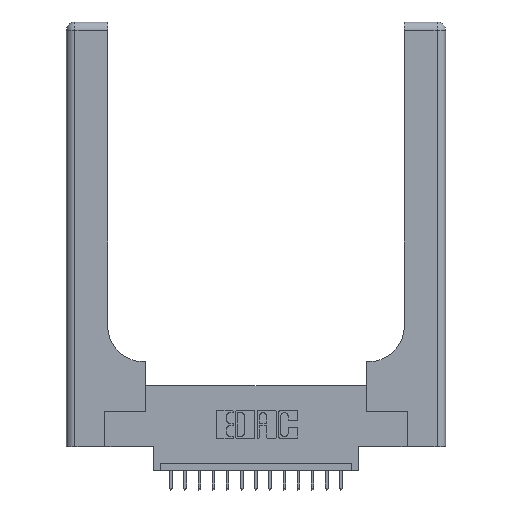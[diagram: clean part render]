
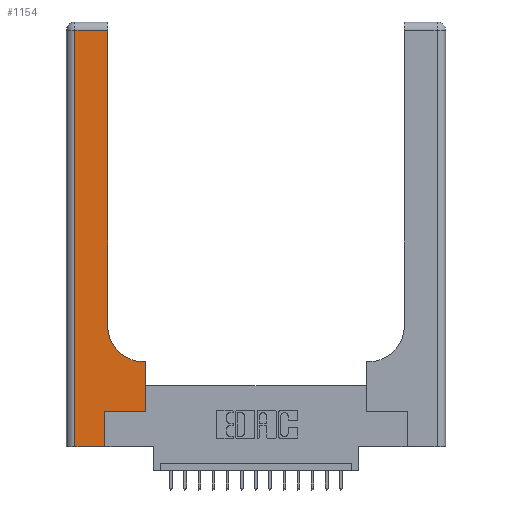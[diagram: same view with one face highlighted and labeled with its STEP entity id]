
A CAD part, top view. The second image highlights one B-rep face of the part: STEP entity #1154.
In plain terms, the highlighted planar face has unit normal (0, 0, 1).
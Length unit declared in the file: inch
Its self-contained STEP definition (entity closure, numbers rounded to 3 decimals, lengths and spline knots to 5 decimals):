
#31 = CARTESIAN_POINT ( 'NONE',  ( 0., 0., 0.37 ) ) ;
#234 = CARTESIAN_POINT ( 'NONE',  ( 0.5585, 0.25, 0.37 ) ) ;
#691 = CARTESIAN_POINT ( 'NONE',  ( 0.06, 3., 0.37 ) ) ;
#1054 = AXIS2_PLACEMENT_3D ( 'NONE', #9260, #11270, #9923 ) ;
#1135 = VERTEX_POINT ( 'NONE', #10544 ) ;
#1154 = ADVANCED_FACE ( 'NONE', ( #6083 ), #12001, .F. ) ;
#1476 = DIRECTION ( 'NONE',  ( -1., 0., 0. ) ) ;
#1492 = ORIENTED_EDGE ( 'NONE', *, *, #18357, .T. ) ;
#1532 = EDGE_CURVE ( 'NONE', #11989, #5757, #1677, .T. ) ;
#1533 = DIRECTION ( 'NONE',  ( -1., 0., 0. ) ) ;
#1605 = VERTEX_POINT ( 'NONE', #7060 ) ;
#1677 = CIRCLE ( 'NONE', #1054, 0.25 ) ;
#2615 = LINE ( 'NONE', #18634, #14400 ) ;
#2927 = LINE ( 'NONE', #31, #18066 ) ;
#3227 = DIRECTION ( 'NONE',  ( 0., 1., 0. ) ) ;
#3379 = CARTESIAN_POINT ( 'NONE',  ( 0.5585, 0.6, 0.37 ) ) ;
#3403 = VERTEX_POINT ( 'NONE', #3379 ) ;
#4426 = VECTOR ( 'NONE', #3227, 39.37008 ) ;
#4508 = CARTESIAN_POINT ( 'NONE',  ( 0.06, 0., 0.37 ) ) ;
#4528 = VECTOR ( 'NONE', #1476, 39.37008 ) ;
#5390 = EDGE_CURVE ( 'NONE', #17710, #1135, #2927, .T. ) ;
#5757 = VERTEX_POINT ( 'NONE', #17192 ) ;
#5866 = LINE ( 'NONE', #234, #4426 ) ;
#6009 = ORIENTED_EDGE ( 'NONE', *, *, #5390, .T. ) ;
#6083 = FACE_OUTER_BOUND ( 'NONE', #13236, .T. ) ;
#6242 = CARTESIAN_POINT ( 'NONE',  ( 0.2915, 3., 0.37 ) ) ;
#6254 = CARTESIAN_POINT ( 'NONE',  ( 0.5415, 0.6, 0.37 ) ) ;
#6740 = DIRECTION ( 'NONE',  ( -1., 0., 0. ) ) ;
#6924 = LINE ( 'NONE', #11186, #15999 ) ;
#7060 = CARTESIAN_POINT ( 'NONE',  ( 0.5585, 0.25, 0.37 ) ) ;
#7928 = EDGE_CURVE ( 'NONE', #17108, #19045, #15490, .T. ) ;
#7969 = EDGE_CURVE ( 'NONE', #1135, #17994, #6924, .T. ) ;
#8840 = CARTESIAN_POINT ( 'NONE',  ( 0.2915, 0.6, 0.37 ) ) ;
#9260 = CARTESIAN_POINT ( 'NONE',  ( 0.5415, 0.85, 0.37 ) ) ;
#9529 = EDGE_CURVE ( 'NONE', #5757, #17108, #12354, .T. ) ;
#9706 = DIRECTION ( 'NONE',  ( 0., -1., 0. ) ) ;
#9779 = ORIENTED_EDGE ( 'NONE', *, *, #7969, .T. ) ;
#9923 = DIRECTION ( 'NONE',  ( 1., 0., 0. ) ) ;
#10032 = ORIENTED_EDGE ( 'NONE', *, *, #10033, .T. ) ;
#10033 = EDGE_CURVE ( 'NONE', #19045, #17710, #15651, .T. ) ;
#10544 = CARTESIAN_POINT ( 'NONE',  ( 0.269, 0., 0.37 ) ) ;
#10791 = VECTOR ( 'NONE', #6740, 39.37008 ) ;
#11186 = CARTESIAN_POINT ( 'NONE',  ( 0.269, 0., 0.37 ) ) ;
#11270 = DIRECTION ( 'NONE',  ( 0., 0., -1. ) ) ;
#11831 = ORIENTED_EDGE ( 'NONE', *, *, #1532, .T. ) ;
#11949 = DIRECTION ( 'NONE',  ( 1., 0., 0. ) ) ;
#11975 = DIRECTION ( 'NONE',  ( 0., 1., 0. ) ) ;
#11989 = VERTEX_POINT ( 'NONE', #6254 ) ;
#12001 = PLANE ( 'NONE',  #16156 ) ;
#12354 = LINE ( 'NONE', #6242, #15687 ) ;
#12386 = EDGE_CURVE ( 'NONE', #1605, #3403, #5866, .T. ) ;
#12811 = CARTESIAN_POINT ( 'NONE',  ( 0.269, 0.25, 0.37 ) ) ;
#12818 = VECTOR ( 'NONE', #9706, 39.37008 ) ;
#13151 = CARTESIAN_POINT ( 'NONE',  ( 0., 3., 0.37 ) ) ;
#13236 = EDGE_LOOP ( 'NONE', ( #16268, #16185, #10032, #6009, #9779, #1492, #16993, #16729, #11831 ) ) ;
#14400 = VECTOR ( 'NONE', #14405, 39.37008 ) ;
#14405 = DIRECTION ( 'NONE',  ( 1., 0., 0. ) ) ;
#15490 = LINE ( 'NONE', #18592, #10791 ) ;
#15565 = CARTESIAN_POINT ( 'NONE',  ( 0.06, 2.94, 0.37 ) ) ;
#15651 = LINE ( 'NONE', #691, #12818 ) ;
#15687 = VECTOR ( 'NONE', #11975, 39.37008 ) ;
#15800 = CARTESIAN_POINT ( 'NONE',  ( 0.2915, 2.94, 0.37 ) ) ;
#15999 = VECTOR ( 'NONE', #17146, 39.37008 ) ;
#16150 = LINE ( 'NONE', #8840, #4528 ) ;
#16156 = AXIS2_PLACEMENT_3D ( 'NONE', #13151, #16212, #1533 ) ;
#16185 = ORIENTED_EDGE ( 'NONE', *, *, #7928, .T. ) ;
#16212 = DIRECTION ( 'NONE',  ( 0., 0., -1. ) ) ;
#16268 = ORIENTED_EDGE ( 'NONE', *, *, #9529, .T. ) ;
#16729 = ORIENTED_EDGE ( 'NONE', *, *, #18151, .T. ) ;
#16993 = ORIENTED_EDGE ( 'NONE', *, *, #12386, .T. ) ;
#17108 = VERTEX_POINT ( 'NONE', #15800 ) ;
#17146 = DIRECTION ( 'NONE',  ( 0., 1., 0. ) ) ;
#17192 = CARTESIAN_POINT ( 'NONE',  ( 0.2915, 0.85, 0.37 ) ) ;
#17710 = VERTEX_POINT ( 'NONE', #4508 ) ;
#17994 = VERTEX_POINT ( 'NONE', #12811 ) ;
#18066 = VECTOR ( 'NONE', #11949, 39.37008 ) ;
#18151 = EDGE_CURVE ( 'NONE', #3403, #11989, #16150, .T. ) ;
#18357 = EDGE_CURVE ( 'NONE', #17994, #1605, #2615, .T. ) ;
#18592 = CARTESIAN_POINT ( 'NONE',  ( 0., 2.94, 0.37 ) ) ;
#18634 = CARTESIAN_POINT ( 'NONE',  ( 0.269, 0.25, 0.37 ) ) ;
#19045 = VERTEX_POINT ( 'NONE', #15565 ) ;
